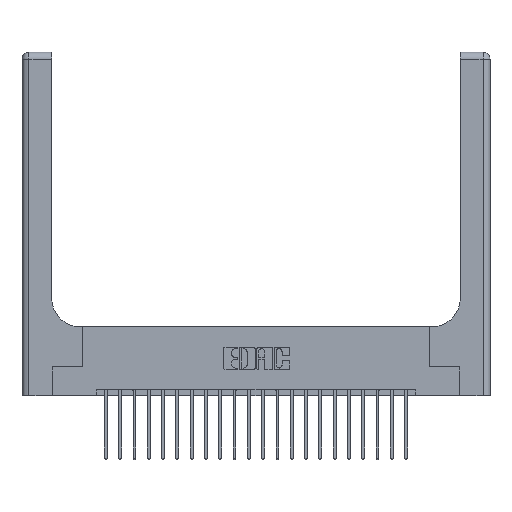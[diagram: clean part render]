
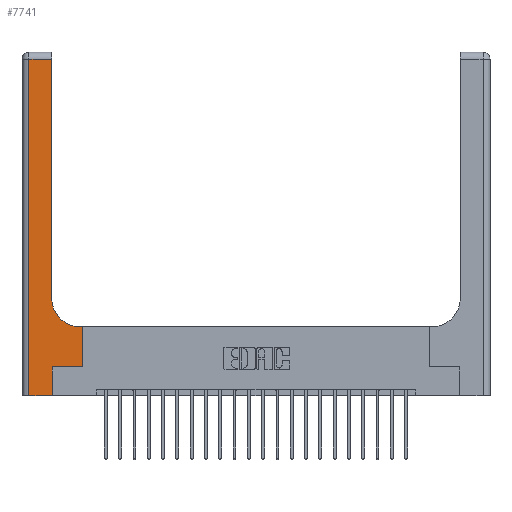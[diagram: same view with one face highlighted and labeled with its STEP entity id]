
A CAD part, top view. The second image highlights one B-rep face of the part: STEP entity #7741.
In plain terms, the highlighted planar face has unit normal (0, 0, 1).
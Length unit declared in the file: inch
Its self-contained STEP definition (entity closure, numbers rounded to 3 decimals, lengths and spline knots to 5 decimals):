
#387 = CARTESIAN_POINT ( 'NONE',  ( 0.265, 0.25, 0.37 ) ) ;
#1137 = LINE ( 'NONE', #18831, #3505 ) ;
#1226 = LINE ( 'NONE', #7998, #6623 ) ;
#1231 = VERTEX_POINT ( 'NONE', #10507 ) ;
#1261 = PLANE ( 'NONE',  #13167 ) ;
#1662 = LINE ( 'NONE', #18912, #2534 ) ;
#2065 = DIRECTION ( 'NONE',  ( 0., 1., 0. ) ) ;
#2213 = DIRECTION ( 'NONE',  ( 0., 1., 0. ) ) ;
#2375 = ORIENTED_EDGE ( 'NONE', *, *, #5492, .T. ) ;
#2534 = VECTOR ( 'NONE', #3161, 39.37008 ) ;
#2698 = LINE ( 'NONE', #387, #19715 ) ;
#3161 = DIRECTION ( 'NONE',  ( 0., -1., 0. ) ) ;
#3314 = CARTESIAN_POINT ( 'NONE',  ( 0.06, 2.94, 0.37 ) ) ;
#3449 = LINE ( 'NONE', #19204, #15161 ) ;
#3505 = VECTOR ( 'NONE', #13757, 39.37008 ) ;
#3560 = CARTESIAN_POINT ( 'NONE',  ( 0.26, 2.94, 0.37 ) ) ;
#3753 = VERTEX_POINT ( 'NONE', #15072 ) ;
#4014 = LINE ( 'NONE', #11267, #18144 ) ;
#4879 = CARTESIAN_POINT ( 'NONE',  ( 0.51, 0.85, 0.37 ) ) ;
#5416 = EDGE_CURVE ( 'NONE', #1231, #10335, #2698, .T. ) ;
#5477 = VERTEX_POINT ( 'NONE', #22315 ) ;
#5492 = EDGE_CURVE ( 'NONE', #6033, #17619, #13527, .T. ) ;
#5550 = VECTOR ( 'NONE', #2213, 39.37008 ) ;
#5640 = LINE ( 'NONE', #12743, #21460 ) ;
#6033 = VERTEX_POINT ( 'NONE', #18535 ) ;
#6196 = EDGE_LOOP ( 'NONE', ( #9731, #21907, #15186, #21115, #15579, #17116, #17105, #7246, #2375 ) ) ;
#6355 = EDGE_CURVE ( 'NONE', #17619, #15503, #4014, .T. ) ;
#6442 = CARTESIAN_POINT ( 'NONE',  ( 0.528, 0.25, 0.37 ) ) ;
#6539 = DIRECTION ( 'NONE',  ( 0., 0., -1. ) ) ;
#6623 = VECTOR ( 'NONE', #14984, 39.37008 ) ;
#7059 = CARTESIAN_POINT ( 'NONE',  ( 0.528, 0.25, 0.37 ) ) ;
#7246 = ORIENTED_EDGE ( 'NONE', *, *, #12506, .T. ) ;
#7741 = ADVANCED_FACE ( 'NONE', ( #17101 ), #1261, .F. ) ;
#7998 = CARTESIAN_POINT ( 'NONE',  ( 0.26, 0.6, 0.37 ) ) ;
#8268 = CARTESIAN_POINT ( 'NONE',  ( 0., 3., 0.37 ) ) ;
#8855 = CARTESIAN_POINT ( 'NONE',  ( 0.528, 0.6, 0.37 ) ) ;
#9493 = CARTESIAN_POINT ( 'NONE',  ( 0.26, 0.85, 0.37 ) ) ;
#9731 = ORIENTED_EDGE ( 'NONE', *, *, #6355, .T. ) ;
#10335 = VERTEX_POINT ( 'NONE', #6442 ) ;
#10507 = CARTESIAN_POINT ( 'NONE',  ( 0.265, 0.25, 0.37 ) ) ;
#10758 = EDGE_CURVE ( 'NONE', #22252, #5477, #1662, .T. ) ;
#10805 = DIRECTION ( 'NONE',  ( 0., 1., 0. ) ) ;
#11267 = CARTESIAN_POINT ( 'NONE',  ( 0.26, 3., 0.37 ) ) ;
#11556 = DIRECTION ( 'NONE',  ( 0., 0., -1. ) ) ;
#12506 = EDGE_CURVE ( 'NONE', #18642, #6033, #1226, .T. ) ;
#12743 = CARTESIAN_POINT ( 'NONE',  ( 0.265, 0., 0.37 ) ) ;
#13167 = AXIS2_PLACEMENT_3D ( 'NONE', #8268, #6539, #13539 ) ;
#13292 = EDGE_CURVE ( 'NONE', #10335, #18642, #17960, .T. ) ;
#13527 = CIRCLE ( 'NONE', #14245, 0.25 ) ;
#13539 = DIRECTION ( 'NONE',  ( -1., 0., 0. ) ) ;
#13757 = DIRECTION ( 'NONE',  ( 1., 0., 0. ) ) ;
#14245 = AXIS2_PLACEMENT_3D ( 'NONE', #4879, #11556, #18782 ) ;
#14406 = DIRECTION ( 'NONE',  ( 1., 0., 0. ) ) ;
#14984 = DIRECTION ( 'NONE',  ( -1., 0., 0. ) ) ;
#15072 = CARTESIAN_POINT ( 'NONE',  ( 0.265, 0., 0.37 ) ) ;
#15161 = VECTOR ( 'NONE', #17471, 39.37008 ) ;
#15186 = ORIENTED_EDGE ( 'NONE', *, *, #10758, .T. ) ;
#15503 = VERTEX_POINT ( 'NONE', #3560 ) ;
#15579 = ORIENTED_EDGE ( 'NONE', *, *, #19964, .T. ) ;
#17101 = FACE_OUTER_BOUND ( 'NONE', #6196, .T. ) ;
#17105 = ORIENTED_EDGE ( 'NONE', *, *, #13292, .T. ) ;
#17116 = ORIENTED_EDGE ( 'NONE', *, *, #5416, .T. ) ;
#17471 = DIRECTION ( 'NONE',  ( -1., 0., 0. ) ) ;
#17619 = VERTEX_POINT ( 'NONE', #9493 ) ;
#17960 = LINE ( 'NONE', #7059, #5550 ) ;
#18144 = VECTOR ( 'NONE', #2065, 39.37008 ) ;
#18535 = CARTESIAN_POINT ( 'NONE',  ( 0.51, 0.6, 0.37 ) ) ;
#18642 = VERTEX_POINT ( 'NONE', #8855 ) ;
#18673 = EDGE_CURVE ( 'NONE', #15503, #22252, #3449, .T. ) ;
#18782 = DIRECTION ( 'NONE',  ( 1., 0., 0. ) ) ;
#18831 = CARTESIAN_POINT ( 'NONE',  ( 0., 0., 0.37 ) ) ;
#18912 = CARTESIAN_POINT ( 'NONE',  ( 0.06, 3., 0.37 ) ) ;
#19204 = CARTESIAN_POINT ( 'NONE',  ( 0., 2.94, 0.37 ) ) ;
#19715 = VECTOR ( 'NONE', #14406, 39.37008 ) ;
#19964 = EDGE_CURVE ( 'NONE', #3753, #1231, #5640, .T. ) ;
#20181 = EDGE_CURVE ( 'NONE', #5477, #3753, #1137, .T. ) ;
#21115 = ORIENTED_EDGE ( 'NONE', *, *, #20181, .T. ) ;
#21460 = VECTOR ( 'NONE', #10805, 39.37008 ) ;
#21907 = ORIENTED_EDGE ( 'NONE', *, *, #18673, .T. ) ;
#22252 = VERTEX_POINT ( 'NONE', #3314 ) ;
#22315 = CARTESIAN_POINT ( 'NONE',  ( 0.06, 0., 0.37 ) ) ;
